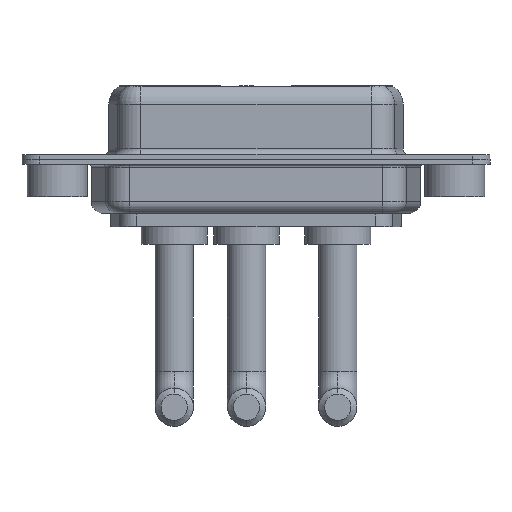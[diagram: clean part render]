
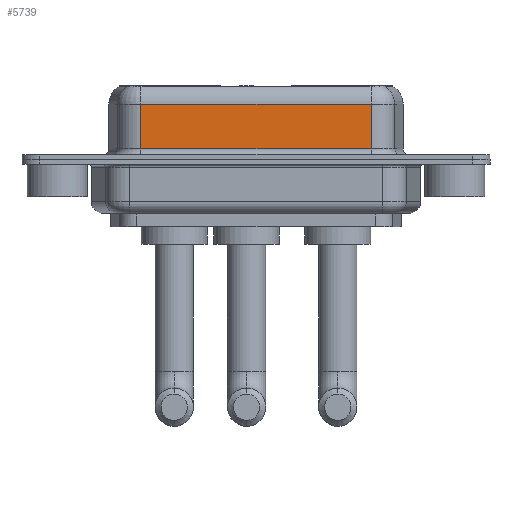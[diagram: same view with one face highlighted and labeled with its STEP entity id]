
A CAD part, front view. The second image highlights one B-rep face of the part: STEP entity #5739.
In plain terms, the highlighted planar face has unit normal (0, -1, 0).
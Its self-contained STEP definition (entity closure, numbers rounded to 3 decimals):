
#46 = EDGE_LOOP ( 'NONE', ( #8981, #7919, #9310, #1830 ) ) ;
#107 = LINE ( 'NONE', #7750, #1350 ) ;
#127 = CARTESIAN_POINT ( 'NONE',  ( 26.287, -3.95, 6.4 ) ) ;
#430 = DIRECTION ( 'NONE',  ( -1., 0., 0. ) ) ;
#472 = VECTOR ( 'NONE', #9531, 1000. ) ;
#1036 = CARTESIAN_POINT ( 'NONE',  ( 26.287, -3.95, 0.9 ) ) ;
#1165 = FACE_OUTER_BOUND ( 'NONE', #46, .T. ) ;
#1350 = VECTOR ( 'NONE', #11027, 1000. ) ;
#1607 = CARTESIAN_POINT ( 'NONE',  ( 26.287, -3.95, 4.65 ) ) ;
#1689 = CARTESIAN_POINT ( 'NONE',  ( 26.287, -3.95, 4.65 ) ) ;
#1830 = ORIENTED_EDGE ( 'NONE', *, *, #4716, .T. ) ;
#3278 = EDGE_CURVE ( 'NONE', #9246, #12728, #11537, .T. ) ;
#3421 = LINE ( 'NONE', #7708, #11128 ) ;
#4261 = CARTESIAN_POINT ( 'NONE',  ( 26.287, -3.95, 6.4 ) ) ;
#4716 = EDGE_CURVE ( 'NONE', #12830, #12728, #3421, .T. ) ;
#5739 = ADVANCED_FACE ( 'NONE', ( #1165 ), #7492, .F. ) ;
#6116 = LINE ( 'NONE', #1689, #10851 ) ;
#6269 = EDGE_CURVE ( 'NONE', #9246, #13581, #6116, .T. ) ;
#6361 = DIRECTION ( 'NONE',  ( 0., 1., 0. ) ) ;
#7492 = PLANE ( 'NONE',  #13020 ) ;
#7708 = CARTESIAN_POINT ( 'NONE',  ( 26.287, -3.95, 0.9 ) ) ;
#7750 = CARTESIAN_POINT ( 'NONE',  ( 7.013, -3.95, 6.4 ) ) ;
#7919 = ORIENTED_EDGE ( 'NONE', *, *, #6269, .T. ) ;
#8981 = ORIENTED_EDGE ( 'NONE', *, *, #3278, .F. ) ;
#9246 = VERTEX_POINT ( 'NONE', #1607 ) ;
#9310 = ORIENTED_EDGE ( 'NONE', *, *, #13275, .T. ) ;
#9531 = DIRECTION ( 'NONE',  ( 0., 0., -1. ) ) ;
#10851 = VECTOR ( 'NONE', #430, 1000. ) ;
#11027 = DIRECTION ( 'NONE',  ( 0., 0., -1. ) ) ;
#11128 = VECTOR ( 'NONE', #11883, 1000. ) ;
#11537 = LINE ( 'NONE', #127, #472 ) ;
#11883 = DIRECTION ( 'NONE',  ( 1., 0., 0. ) ) ;
#12705 = CARTESIAN_POINT ( 'NONE',  ( 7.013, -3.95, 4.65 ) ) ;
#12728 = VERTEX_POINT ( 'NONE', #1036 ) ;
#12830 = VERTEX_POINT ( 'NONE', #13059 ) ;
#12915 = DIRECTION ( 'NONE',  ( 0., 0., 1. ) ) ;
#13020 = AXIS2_PLACEMENT_3D ( 'NONE', #4261, #6361, #12915 ) ;
#13059 = CARTESIAN_POINT ( 'NONE',  ( 7.013, -3.95, 0.9 ) ) ;
#13275 = EDGE_CURVE ( 'NONE', #13581, #12830, #107, .T. ) ;
#13581 = VERTEX_POINT ( 'NONE', #12705 ) ;
